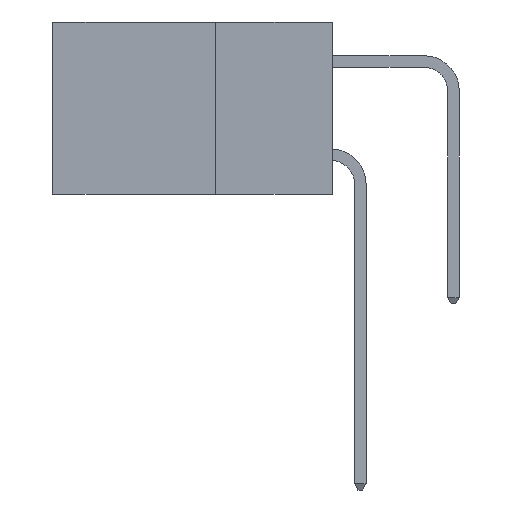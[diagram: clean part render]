
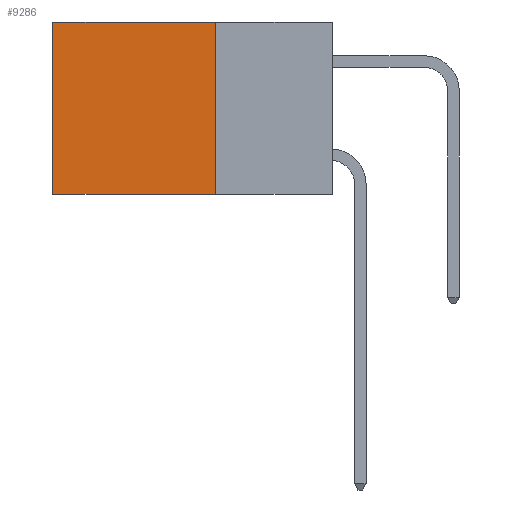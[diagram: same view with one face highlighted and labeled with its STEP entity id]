
A CAD part, left-side view. The second image highlights one B-rep face of the part: STEP entity #9286.
In plain terms, the highlighted planar face has unit normal (-1, 0, 0).
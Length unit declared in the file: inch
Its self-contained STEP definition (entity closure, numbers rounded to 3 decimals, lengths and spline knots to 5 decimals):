
#61 = EDGE_CURVE ( 'NONE', #8351, #9479, #2427, .T. ) ;
#1422 = FACE_OUTER_BOUND ( 'NONE', #7230, .T. ) ;
#1963 = VECTOR ( 'NONE', #13006, 39.37008 ) ;
#1998 = LINE ( 'NONE', #10446, #2624 ) ;
#2427 = LINE ( 'NONE', #11922, #1963 ) ;
#2624 = VECTOR ( 'NONE', #9368, 39.37008 ) ;
#3072 = LINE ( 'NONE', #5565, #11004 ) ;
#3676 = CARTESIAN_POINT ( 'NONE',  ( 0.2615, 0.25, -0.37 ) ) ;
#4158 = CARTESIAN_POINT ( 'NONE',  ( 0.2615, 0.25, 0. ) ) ;
#4171 = DIRECTION ( 'NONE',  ( 0., 1., 0. ) ) ;
#4265 = VERTEX_POINT ( 'NONE', #3676 ) ;
#4396 = AXIS2_PLACEMENT_3D ( 'NONE', #8174, #10351, #7365 ) ;
#4999 = CARTESIAN_POINT ( 'NONE',  ( 0.2615, 0.25, -0.37 ) ) ;
#5283 = EDGE_CURVE ( 'NONE', #4265, #12948, #7526, .T. ) ;
#5382 = EDGE_CURVE ( 'NONE', #9479, #12948, #1998, .T. ) ;
#5565 = CARTESIAN_POINT ( 'NONE',  ( 0.2615, 0.25, -0.37 ) ) ;
#5965 = PLANE ( 'NONE',  #4396 ) ;
#6140 = VECTOR ( 'NONE', #4171, 39.37008 ) ;
#7230 = EDGE_LOOP ( 'NONE', ( #10682, #10221, #8942, #7381 ) ) ;
#7365 = DIRECTION ( 'NONE',  ( 0., 0., -1. ) ) ;
#7381 = ORIENTED_EDGE ( 'NONE', *, *, #61, .T. ) ;
#7526 = LINE ( 'NONE', #4999, #6140 ) ;
#7571 = CARTESIAN_POINT ( 'NONE',  ( 0.2615, 0.6, 0. ) ) ;
#7593 = CARTESIAN_POINT ( 'NONE',  ( 0.2615, 0.6, -0.37 ) ) ;
#8174 = CARTESIAN_POINT ( 'NONE',  ( 0.2615, 0.25, -0.37 ) ) ;
#8351 = VERTEX_POINT ( 'NONE', #4158 ) ;
#8942 = ORIENTED_EDGE ( 'NONE', *, *, #11834, .F. ) ;
#9286 = ADVANCED_FACE ( 'NONE', ( #1422 ), #5965, .F. ) ;
#9368 = DIRECTION ( 'NONE',  ( 0., 0., -1. ) ) ;
#9479 = VERTEX_POINT ( 'NONE', #7571 ) ;
#10221 = ORIENTED_EDGE ( 'NONE', *, *, #5283, .F. ) ;
#10351 = DIRECTION ( 'NONE',  ( 1., 0., 0. ) ) ;
#10446 = CARTESIAN_POINT ( 'NONE',  ( 0.2615, 0.6, -0.37 ) ) ;
#10682 = ORIENTED_EDGE ( 'NONE', *, *, #5382, .T. ) ;
#11004 = VECTOR ( 'NONE', #11588, 39.37008 ) ;
#11588 = DIRECTION ( 'NONE',  ( 0., 0., -1. ) ) ;
#11834 = EDGE_CURVE ( 'NONE', #8351, #4265, #3072, .T. ) ;
#11922 = CARTESIAN_POINT ( 'NONE',  ( 0.2615, 0.25, 0. ) ) ;
#12948 = VERTEX_POINT ( 'NONE', #7593 ) ;
#13006 = DIRECTION ( 'NONE',  ( 0., 1., 0. ) ) ;
